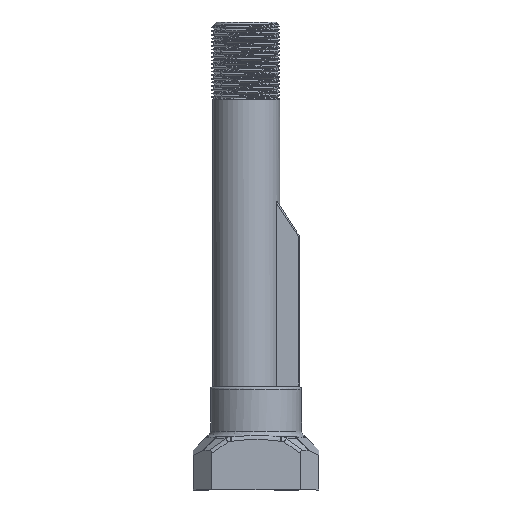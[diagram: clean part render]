
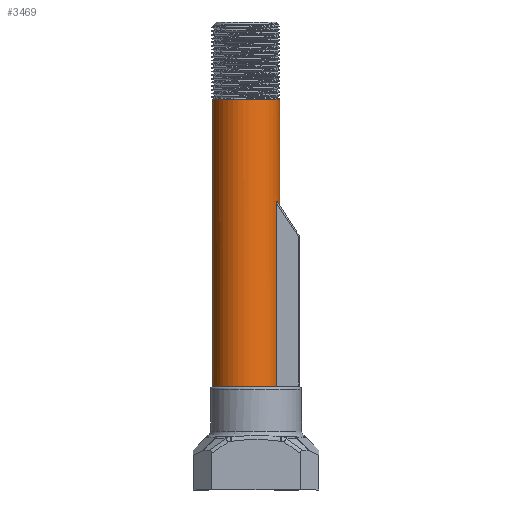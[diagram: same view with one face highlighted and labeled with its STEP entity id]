
A CAD part, left-side view. The second image highlights one B-rep face of the part: STEP entity #3469.
In plain terms, the highlighted cylindrical face has radius 14.5 mm (diameter 29 mm), a full revolution.
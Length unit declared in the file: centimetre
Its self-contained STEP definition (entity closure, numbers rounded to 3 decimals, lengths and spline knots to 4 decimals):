
#44=ELLIPSE($,#3733,2.6293,1.45);
#201=B_SPLINE_CURVE_WITH_KNOTS($,3,(#9700,#9701,#9702,#9703,#9704,#9705,
#9706,#9707,#9708,#9709,#9710,#9711,#9712,#9713,#9714,#9715),
 .UNSPECIFIED.,.F.,.F.,(4,2,2,2,2,2,2,4),(0.361,0.3719,
0.3827,0.392,0.4013,0.4152,
0.4291,0.4569),.UNSPECIFIED.);
#202=B_SPLINE_CURVE_WITH_KNOTS($,3,(#9719,#9720,#9721,#9722,#9723,#9724,
#9725,#9726,#9727,#9728,#9729,#9730,#9731,#9732,#9733,#9734),
 .UNSPECIFIED.,.F.,.F.,(4,2,2,2,2,2,2,4),(0.,0.0278,
0.0417,0.0556,0.0649,0.0741,
0.085,0.0958),.UNSPECIFIED.);
#374=FACE_BOUND($,#724,.T.);
#512=FACE_OUTER_BOUND($,#723,.T.);
#723=EDGE_LOOP($,(#2572,#2573,#2574,#2575,#2576,#2577));
#724=EDGE_LOOP($,(#2578,#2579));
#911=LINE($,#4909,#1073);
#912=LINE($,#9735,#1074);
#1073=VECTOR($,#4149,12.3693);
#1074=VECTOR($,#4202,12.3693);
#1239=CIRCLE($,#3695,1.45);
#1254=CIRCLE($,#3731,1.45);
#1255=CIRCLE($,#3734,1.45);
#1372=VERTEX_POINT($,#4880);
#1373=VERTEX_POINT($,#4882);
#1378=VERTEX_POINT($,#4907);
#1487=VERTEX_POINT($,#9641);
#1488=VERTEX_POINT($,#9660);
#1489=VERTEX_POINT($,#9699);
#1490=VERTEX_POINT($,#9716);
#1491=VERTEX_POINT($,#9718);
#1791=EDGE_CURVE($,#1373,#1372,#1239,.T.);
#1805=EDGE_CURVE($,#1378,#1372,#911,.T.);
#1918=EDGE_CURVE($,#1487,#1488,#1254,.T.);
#1919=EDGE_CURVE($,#1378,#1489,#201,.F.);
#1920=EDGE_CURVE($,#1490,#1489,#44,.T.);
#1921=EDGE_CURVE($,#1490,#1491,#202,.F.);
#1922=EDGE_CURVE($,#1373,#1491,#912,.T.);
#1923=EDGE_CURVE($,#1488,#1487,#1255,.T.);
#2572=ORIENTED_EDGE($,*,*,#1791,.T.);
#2573=ORIENTED_EDGE($,*,*,#1805,.F.);
#2574=ORIENTED_EDGE($,*,*,#1919,.T.);
#2575=ORIENTED_EDGE($,*,*,#1920,.F.);
#2576=ORIENTED_EDGE($,*,*,#1921,.T.);
#2577=ORIENTED_EDGE($,*,*,#1922,.F.);
#2578=ORIENTED_EDGE($,*,*,#1918,.T.);
#2579=ORIENTED_EDGE($,*,*,#1923,.T.);
#3387=CYLINDRICAL_SURFACE($,#3732,1.45);
#3469=ADVANCED_FACE($,(#512,#374),#3387,.T.);
#3695=AXIS2_PLACEMENT_3D($,#4883,#4115,#4116);
#3731=AXIS2_PLACEMENT_3D($,#9697,#4196,#4197);
#3732=AXIS2_PLACEMENT_3D($,#9698,#4198,#4199);
#3733=AXIS2_PLACEMENT_3D($,#9717,#4200,#4201);
#3734=AXIS2_PLACEMENT_3D($,#9736,#4203,#4204);
#4115=DIRECTION('center_axis',(0.,0.,1.));
#4116=DIRECTION('ref_axis',(-1.,0.,0.));
#4149=DIRECTION($,(0.,0.,-1.));
#4196=DIRECTION('center_axis',(0.,0.,-1.));
#4197=DIRECTION('ref_axis',(-1.,0.,0.));
#4198=DIRECTION('center_axis',(0.,0.,1.));
#4199=DIRECTION('ref_axis',(-1.,0.,0.));
#4200=DIRECTION('center_axis',(0.,0.834,
-0.551));
#4201=DIRECTION('ref_axis',(0.,-0.551,-0.834));
#4202=DIRECTION($,(0.,0.,1.));
#4203=DIRECTION('center_axis',(0.,0.,-1.));
#4204=DIRECTION('ref_axis',(-1.,0.,0.));
#4880=CARTESIAN_POINT('',(-17.625,24.6107,2.04));
#4882=CARTESIAN_POINT('',(-16.375,24.6107,2.04));
#4883=CARTESIAN_POINT('Origin',(-17.,25.9191,2.04));
#4907=CARTESIAN_POINT('',(-17.625,24.6107,14.4093));
#4909=CARTESIAN_POINT($,(-17.625,24.6107,15.));
#9641=CARTESIAN_POINT('',(-18.2063,26.7238,18.9));
#9660=CARTESIAN_POINT('',(-17.4557,24.5426,18.9));
#9697=CARTESIAN_POINT('Origin',(-17.,25.9191,18.9));
#9698=CARTESIAN_POINT('Origin',(-17.,25.9191,15.));
#9699=CARTESIAN_POINT('',(-17.575,24.588,14.4656));
#9700=CARTESIAN_POINT('Ctrl Pts',(-17.575,24.588,14.4656));
#9701=CARTESIAN_POINT('Ctrl Pts',(-17.5778,24.5892,14.4675));
#9702=CARTESIAN_POINT('Ctrl Pts',(-17.5811,24.5907,14.4692));
#9703=CARTESIAN_POINT('Ctrl Pts',(-17.588,24.5937,14.4713));
#9704=CARTESIAN_POINT('Ctrl Pts',(-17.5915,24.5953,14.4717));
#9705=CARTESIAN_POINT('Ctrl Pts',(-17.5976,24.598,14.4711));
#9706=CARTESIAN_POINT('Ctrl Pts',(-17.6006,24.5993,14.4702));
#9707=CARTESIAN_POINT('Ctrl Pts',(-17.6059,24.6018,14.4673));
#9708=CARTESIAN_POINT('Ctrl Pts',(-17.6084,24.6029,14.4652));
#9709=CARTESIAN_POINT('Ctrl Pts',(-17.6133,24.6052,14.4597));
#9710=CARTESIAN_POINT('Ctrl Pts',(-17.6156,24.6063,14.4559));
#9711=CARTESIAN_POINT('Ctrl Pts',(-17.6194,24.6081,14.4474));
#9712=CARTESIAN_POINT('Ctrl Pts',(-17.6209,24.6088,14.4429));
#9713=CARTESIAN_POINT('Ctrl Pts',(-17.6242,24.6104,14.4287));
#9714=CARTESIAN_POINT('Ctrl Pts',(-17.625,24.6107,14.4186));
#9715=CARTESIAN_POINT('Ctrl Pts',(-17.625,24.6107,14.4093));
#9716=CARTESIAN_POINT('',(-16.425,24.588,14.4656));
#9717=CARTESIAN_POINT('Origin',(-17.,25.9191,16.4792));
#9718=CARTESIAN_POINT('',(-16.375,24.6107,14.4093));
#9719=CARTESIAN_POINT('Ctrl Pts',(-16.375,24.6107,14.4093));
#9720=CARTESIAN_POINT('Ctrl Pts',(-16.375,24.6107,14.4186));
#9721=CARTESIAN_POINT('Ctrl Pts',(-16.3758,24.6104,14.4287));
#9722=CARTESIAN_POINT('Ctrl Pts',(-16.3791,24.6088,14.4429));
#9723=CARTESIAN_POINT('Ctrl Pts',(-16.3806,24.6081,14.4474));
#9724=CARTESIAN_POINT('Ctrl Pts',(-16.3844,24.6063,14.4559));
#9725=CARTESIAN_POINT('Ctrl Pts',(-16.3867,24.6052,14.4597));
#9726=CARTESIAN_POINT('Ctrl Pts',(-16.3916,24.6029,14.4652));
#9727=CARTESIAN_POINT('Ctrl Pts',(-16.3941,24.6018,14.4673));
#9728=CARTESIAN_POINT('Ctrl Pts',(-16.3994,24.5993,14.4702));
#9729=CARTESIAN_POINT('Ctrl Pts',(-16.4024,24.598,14.4711));
#9730=CARTESIAN_POINT('Ctrl Pts',(-16.4085,24.5953,14.4717));
#9731=CARTESIAN_POINT('Ctrl Pts',(-16.412,24.5937,14.4713));
#9732=CARTESIAN_POINT('Ctrl Pts',(-16.4189,24.5907,14.4692));
#9733=CARTESIAN_POINT('Ctrl Pts',(-16.4222,24.5892,14.4675));
#9734=CARTESIAN_POINT('Ctrl Pts',(-16.425,24.588,14.4656));
#9735=CARTESIAN_POINT($,(-16.375,24.6107,15.));
#9736=CARTESIAN_POINT('Origin',(-17.,25.9191,18.9));
